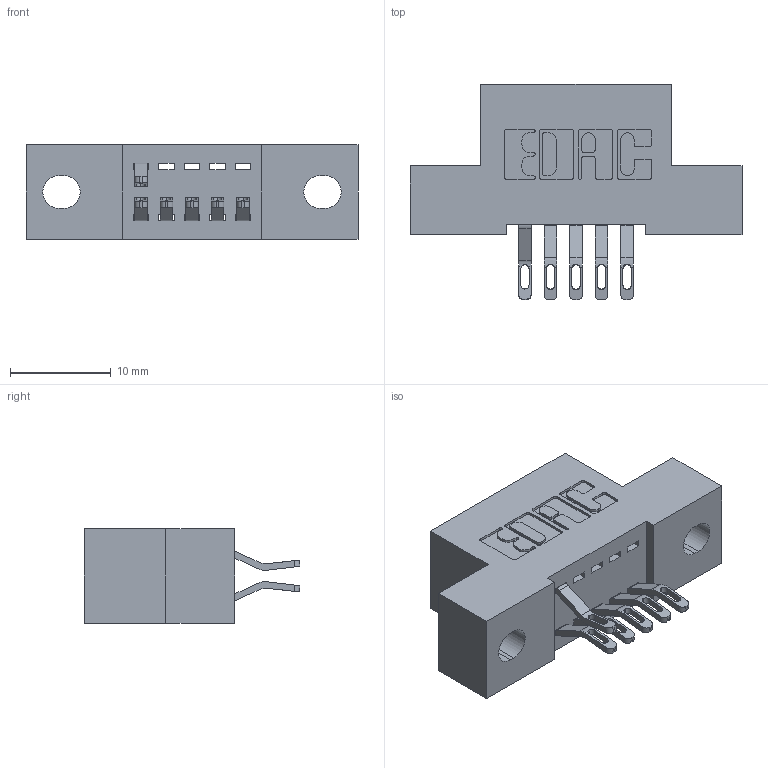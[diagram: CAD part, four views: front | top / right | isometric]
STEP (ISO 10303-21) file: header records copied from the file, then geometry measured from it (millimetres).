
FILE_DESCRIPTION (( 'STEP AP203' ), '1' );
FILE_NAME ('342-010-555-202.STEP', '2018-08-10T13:53:10', ( '' ), ( '' ), 'SwSTEP 2.0', 'SolidWorks 2016', '' );
FILE_SCHEMA (( 'CONFIG_CONTROL_DESIGN' ));
Length unit declared in the file: inch
Products named in the file (3): 342 Part_.128 Slot; 345-292-001_555 Tail; 342-010-555-202
Assembly tree (7 placements, depth 2):
  342-010-555-202
    342 Part_.128 Slot
    345-292-001_555 Tail  x6
Bounding box: 33.02 x 21.47 x 9.4 mm (x, y, z)
Volume: 2720.2 mm3; surface area: 3134.8 mm2
Topology: 7 solids, 7 shells, 486 faces, 1493 edges, 994 vertices
Faces by surface type: plane 298, cylinder 188
Entity records: 8203 total; most frequent: CARTESIAN_POINT 1456, ORIENTED_EDGE 1366, DIRECTION 1275, EDGE_CURVE 683, VECTOR 535, LINE 535, VERTEX_POINT 454, AXIS2_PLACEMENT_3D 370
